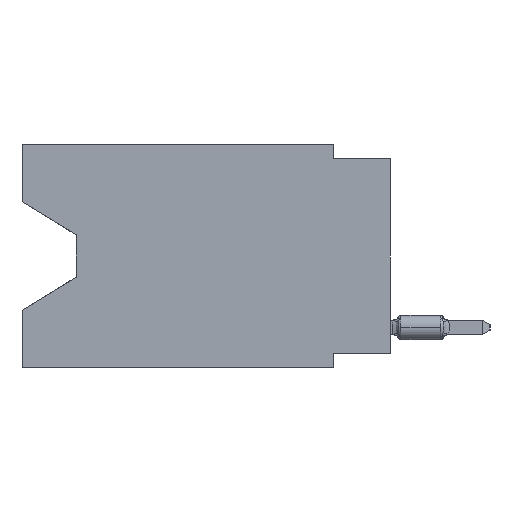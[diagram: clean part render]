
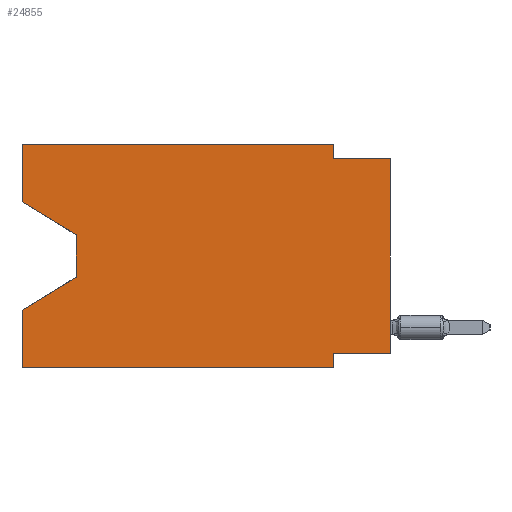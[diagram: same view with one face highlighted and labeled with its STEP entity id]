
A CAD part, left-side view. The second image highlights one B-rep face of the part: STEP entity #24855.
In plain terms, the highlighted planar face has unit normal (-1, 0, 0).
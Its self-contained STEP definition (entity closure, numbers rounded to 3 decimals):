
#203 = VECTOR ( 'NONE', #2938, 1000. ) ;
#244 = VERTEX_POINT ( 'NONE', #21560 ) ;
#253 = LINE ( 'NONE', #31503, #31039 ) ;
#675 = CARTESIAN_POINT ( 'NONE',  ( 0., 0., -9.271 ) ) ;
#1124 = ORIENTED_EDGE ( 'NONE', *, *, #30319, .T. ) ;
#1930 = CARTESIAN_POINT ( 'NONE',  ( 0., 2.54, 0. ) ) ;
#2123 = CARTESIAN_POINT ( 'NONE',  ( 0., 16.383, 0. ) ) ;
#2322 = LINE ( 'NONE', #24429, #6687 ) ;
#2549 = LINE ( 'NONE', #31332, #27890 ) ;
#2938 = DIRECTION ( 'NONE',  ( 0., 0., 1. ) ) ;
#2956 = DIRECTION ( 'NONE',  ( 0., -1., 0. ) ) ;
#3203 = ORIENTED_EDGE ( 'NONE', *, *, #12261, .F. ) ;
#3509 = VECTOR ( 'NONE', #12428, 1000. ) ;
#4135 = ORIENTED_EDGE ( 'NONE', *, *, #38662, .T. ) ;
#5829 = EDGE_CURVE ( 'NONE', #42626, #19931, #15155, .T. ) ;
#6398 = LINE ( 'NONE', #17090, #14805 ) ;
#6687 = VECTOR ( 'NONE', #10377, 1000. ) ;
#7471 = DIRECTION ( 'NONE',  ( 0., -1., 0. ) ) ;
#8125 = AXIS2_PLACEMENT_3D ( 'NONE', #31996, #26834, #37560 ) ;
#8640 = CARTESIAN_POINT ( 'NONE',  ( 0., 16.383, -9.906 ) ) ;
#9565 = VERTEX_POINT ( 'NONE', #33598 ) ;
#9624 = CARTESIAN_POINT ( 'NONE',  ( 0., 13.97, -4.013 ) ) ;
#9842 = LINE ( 'NONE', #24355, #40080 ) ;
#10377 = DIRECTION ( 'NONE',  ( 0., 0., -1. ) ) ;
#10834 = DIRECTION ( 'NONE',  ( 0., -0.855, -0.519 ) ) ;
#11123 = DIRECTION ( 'NONE',  ( 0., 1., 0. ) ) ;
#11787 = VERTEX_POINT ( 'NONE', #36133 ) ;
#12261 = EDGE_CURVE ( 'NONE', #17167, #29384, #19561, .T. ) ;
#12428 = DIRECTION ( 'NONE',  ( 0., 0., 1. ) ) ;
#12583 = EDGE_CURVE ( 'NONE', #41821, #244, #25467, .T. ) ;
#12843 = EDGE_LOOP ( 'NONE', ( #13884, #30515, #1124, #3203, #4135, #19879, #40791, #23499, #19249, #33926, #32487, #46345 ) ) ;
#13271 = CARTESIAN_POINT ( 'NONE',  ( 0., 0., -9.271 ) ) ;
#13549 = EDGE_CURVE ( 'NONE', #45978, #17176, #2549, .T. ) ;
#13884 = ORIENTED_EDGE ( 'NONE', *, *, #14961, .T. ) ;
#14101 = EDGE_CURVE ( 'NONE', #17176, #9565, #9842, .T. ) ;
#14805 = VECTOR ( 'NONE', #35436, 1000. ) ;
#14961 = EDGE_CURVE ( 'NONE', #15268, #41821, #32978, .T. ) ;
#15155 = LINE ( 'NONE', #675, #17479 ) ;
#15268 = VERTEX_POINT ( 'NONE', #17786 ) ;
#16305 = CARTESIAN_POINT ( 'NONE',  ( 0., 16.383, 0. ) ) ;
#17090 = CARTESIAN_POINT ( 'NONE',  ( 0., 16.383, -9.906 ) ) ;
#17167 = VERTEX_POINT ( 'NONE', #8640 ) ;
#17176 = VERTEX_POINT ( 'NONE', #34581 ) ;
#17457 = FACE_OUTER_BOUND ( 'NONE', #12843, .T. ) ;
#17479 = VECTOR ( 'NONE', #11123, 1000. ) ;
#17786 = CARTESIAN_POINT ( 'NONE',  ( 0., 16.383, -2.546 ) ) ;
#19249 = ORIENTED_EDGE ( 'NONE', *, *, #14101, .F. ) ;
#19561 = LINE ( 'NONE', #41468, #3509 ) ;
#19879 = ORIENTED_EDGE ( 'NONE', *, *, #28300, .F. ) ;
#19931 = VERTEX_POINT ( 'NONE', #34064 ) ;
#21560 = CARTESIAN_POINT ( 'NONE',  ( 0., 13.97, -5.893 ) ) ;
#22240 = VECTOR ( 'NONE', #45360, 1000. ) ;
#23499 = ORIENTED_EDGE ( 'NONE', *, *, #43575, .T. ) ;
#24248 = CARTESIAN_POINT ( 'NONE',  ( 0., 16.383, -2.546 ) ) ;
#24355 = CARTESIAN_POINT ( 'NONE',  ( 0., 0., -0.635 ) ) ;
#24429 = CARTESIAN_POINT ( 'NONE',  ( 0., 2.54, -9.906 ) ) ;
#24855 = ADVANCED_FACE ( 'NONE', ( #17457 ), #39148, .F. ) ;
#25258 = LINE ( 'NONE', #39806, #203 ) ;
#25467 = LINE ( 'NONE', #33104, #39267 ) ;
#26834 = DIRECTION ( 'NONE',  ( 1., 0., 0. ) ) ;
#27890 = VECTOR ( 'NONE', #41815, 1000. ) ;
#28300 = EDGE_CURVE ( 'NONE', #19931, #11787, #2322, .T. ) ;
#29384 = VERTEX_POINT ( 'NONE', #45208 ) ;
#30319 = EDGE_CURVE ( 'NONE', #244, #29384, #253, .T. ) ;
#30515 = ORIENTED_EDGE ( 'NONE', *, *, #12583, .T. ) ;
#30808 = VECTOR ( 'NONE', #7471, 1000. ) ;
#31039 = VECTOR ( 'NONE', #46891, 1000. ) ;
#31332 = CARTESIAN_POINT ( 'NONE',  ( 0., 2.54, 0. ) ) ;
#31503 = CARTESIAN_POINT ( 'NONE',  ( 0., 13.97, -5.893 ) ) ;
#31996 = CARTESIAN_POINT ( 'NONE',  ( 0., 16.383, 0. ) ) ;
#32487 = ORIENTED_EDGE ( 'NONE', *, *, #38320, .F. ) ;
#32978 = LINE ( 'NONE', #24248, #37893 ) ;
#33104 = CARTESIAN_POINT ( 'NONE',  ( 0., 13.97, -4.013 ) ) ;
#33178 = LINE ( 'NONE', #36510, #30808 ) ;
#33598 = CARTESIAN_POINT ( 'NONE',  ( 0., 0., -0.635 ) ) ;
#33926 = ORIENTED_EDGE ( 'NONE', *, *, #13549, .F. ) ;
#34064 = CARTESIAN_POINT ( 'NONE',  ( 0., 2.54, -9.271 ) ) ;
#34581 = CARTESIAN_POINT ( 'NONE',  ( 0., 2.54, -0.635 ) ) ;
#35125 = LINE ( 'NONE', #16305, #22240 ) ;
#35427 = EDGE_CURVE ( 'NONE', #15268, #43695, #35125, .T. ) ;
#35436 = DIRECTION ( 'NONE',  ( 0., -1., 0. ) ) ;
#36133 = CARTESIAN_POINT ( 'NONE',  ( 0., 2.54, -9.906 ) ) ;
#36510 = CARTESIAN_POINT ( 'NONE',  ( 0., 16.383, 0. ) ) ;
#37560 = DIRECTION ( 'NONE',  ( 0., 0., -1. ) ) ;
#37893 = VECTOR ( 'NONE', #10834, 1000. ) ;
#38320 = EDGE_CURVE ( 'NONE', #43695, #45978, #33178, .T. ) ;
#38662 = EDGE_CURVE ( 'NONE', #17167, #11787, #6398, .T. ) ;
#39148 = PLANE ( 'NONE',  #8125 ) ;
#39267 = VECTOR ( 'NONE', #44289, 1000. ) ;
#39806 = CARTESIAN_POINT ( 'NONE',  ( 0., 0., 0. ) ) ;
#40080 = VECTOR ( 'NONE', #2956, 1000. ) ;
#40791 = ORIENTED_EDGE ( 'NONE', *, *, #5829, .F. ) ;
#41468 = CARTESIAN_POINT ( 'NONE',  ( 0., 16.383, 0. ) ) ;
#41815 = DIRECTION ( 'NONE',  ( 0., 0., -1. ) ) ;
#41821 = VERTEX_POINT ( 'NONE', #9624 ) ;
#42626 = VERTEX_POINT ( 'NONE', #13271 ) ;
#43575 = EDGE_CURVE ( 'NONE', #42626, #9565, #25258, .T. ) ;
#43695 = VERTEX_POINT ( 'NONE', #2123 ) ;
#44289 = DIRECTION ( 'NONE',  ( 0., 0., -1. ) ) ;
#45208 = CARTESIAN_POINT ( 'NONE',  ( 0., 16.383, -7.36 ) ) ;
#45360 = DIRECTION ( 'NONE',  ( 0., 0., 1. ) ) ;
#45978 = VERTEX_POINT ( 'NONE', #1930 ) ;
#46345 = ORIENTED_EDGE ( 'NONE', *, *, #35427, .F. ) ;
#46891 = DIRECTION ( 'NONE',  ( 0., 0.855, -0.519 ) ) ;
